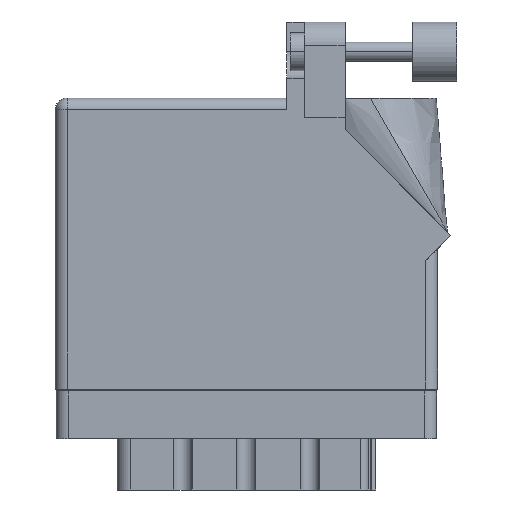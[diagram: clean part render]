
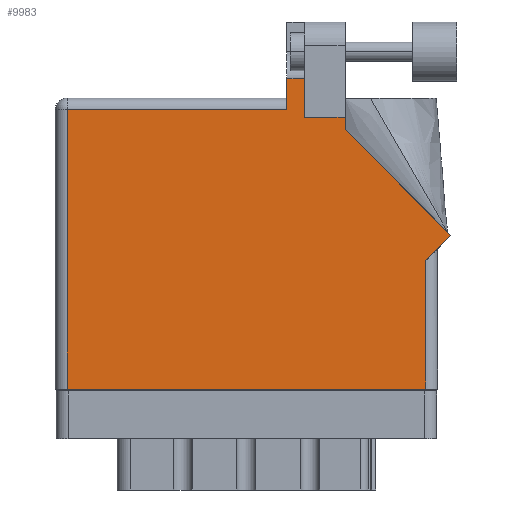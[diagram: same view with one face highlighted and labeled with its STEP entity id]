
A CAD part, front view. The second image highlights one B-rep face of the part: STEP entity #9983.
In plain terms, the highlighted face is planar.
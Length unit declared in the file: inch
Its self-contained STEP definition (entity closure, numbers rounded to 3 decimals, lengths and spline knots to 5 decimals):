
#155 = LINE ( 'NONE', #9917, #4669 ) ;
#1623 = EDGE_CURVE ( 'NONE', #24124, #27353, #11907, .T. ) ;
#1739 = DIRECTION ( 'NONE',  ( -1., 0., 0. ) ) ;
#1949 = CARTESIAN_POINT ( 'NONE',  ( 1.948, 0.675, 0. ) ) ;
#1974 = LINE ( 'NONE', #24542, #31840 ) ;
#2134 = PLANE ( 'NONE',  #11080 ) ;
#3184 = EDGE_CURVE ( 'NONE', #17469, #32814, #34057, .T. ) ;
#3371 = ORIENTED_EDGE ( 'NONE', *, *, #4933, .T. ) ;
#3583 = VECTOR ( 'NONE', #19565, 39.37008 ) ;
#3802 = VERTEX_POINT ( 'NONE', #10859 ) ;
#3973 = DIRECTION ( 'NONE',  ( 0.707, 0.707, 0. ) ) ;
#4469 = VERTEX_POINT ( 'NONE', #26020 ) ;
#4598 = VERTEX_POINT ( 'NONE', #9753 ) ;
#4600 = ORIENTED_EDGE ( 'NONE', *, *, #5607, .T. ) ;
#4647 = FACE_OUTER_BOUND ( 'NONE', #32032, .T. ) ;
#4669 = VECTOR ( 'NONE', #15663, 39.37008 ) ;
#4933 = EDGE_CURVE ( 'NONE', #27353, #31644, #31674, .T. ) ;
#5364 = EDGE_CURVE ( 'NONE', #24194, #23527, #28900, .T. ) ;
#5607 = EDGE_CURVE ( 'NONE', #31644, #24194, #9808, .T. ) ;
#5779 = VECTOR ( 'NONE', #32070, 39.37008 ) ;
#6539 = EDGE_CURVE ( 'NONE', #4469, #24124, #32995, .T. ) ;
#7675 = CARTESIAN_POINT ( 'NONE',  ( 1.948, 0., 0. ) ) ;
#7833 = CARTESIAN_POINT ( 'NONE',  ( 1.524, 1.36442, 0. ) ) ;
#8249 = DIRECTION ( 'NONE',  ( -1., 0., 0. ) ) ;
#8918 = CARTESIAN_POINT ( 'NONE',  ( 2.08071, 0.80771, 0. ) ) ;
#9753 = CARTESIAN_POINT ( 'NONE',  ( 1.311, 1.43, 0. ) ) ;
#9808 = LINE ( 'NONE', #35729, #22561 ) ;
#9860 = ORIENTED_EDGE ( 'NONE', *, *, #5364, .T. ) ;
#9882 = CARTESIAN_POINT ( 'NONE',  ( 1.217, 1.468, 0. ) ) ;
#9917 = CARTESIAN_POINT ( 'NONE',  ( 1.311, 1.43, 0. ) ) ;
#9983 = ADVANCED_FACE ( 'NONE', ( #4647 ), #2134, .F. ) ;
#10069 = EDGE_CURVE ( 'NONE', #3802, #17469, #23673, .T. ) ;
#10307 = CARTESIAN_POINT ( 'NONE',  ( 1.524, 1.36442, 0. ) ) ;
#10434 = DIRECTION ( 'NONE',  ( -1., 0., 0. ) ) ;
#10859 = CARTESIAN_POINT ( 'NONE',  ( 1.311, 1.6315, 0. ) ) ;
#10913 = CARTESIAN_POINT ( 'NONE',  ( 1.948, 0.737, 0. ) ) ;
#11080 = AXIS2_PLACEMENT_3D ( 'NONE', #22373, #34245, #8249 ) ;
#11907 = LINE ( 'NONE', #16875, #28661 ) ;
#12183 = VERTEX_POINT ( 'NONE', #17474 ) ;
#13902 = ORIENTED_EDGE ( 'NONE', *, *, #29931, .T. ) ;
#14815 = ORIENTED_EDGE ( 'NONE', *, *, #30037, .T. ) ;
#15663 = DIRECTION ( 'NONE',  ( 0., 1., 0. ) ) ;
#15686 = CARTESIAN_POINT ( 'NONE',  ( 1.217, 1.53, 0. ) ) ;
#15942 = DIRECTION ( 'NONE',  ( 0., -1., 0. ) ) ;
#16422 = VECTOR ( 'NONE', #15942, 39.37008 ) ;
#16875 = CARTESIAN_POINT ( 'NONE',  ( 0., 0., 0. ) ) ;
#17087 = ORIENTED_EDGE ( 'NONE', *, *, #3184, .T. ) ;
#17469 = VERTEX_POINT ( 'NONE', #37457 ) ;
#17474 = CARTESIAN_POINT ( 'NONE',  ( 1.524, 1.43, 0. ) ) ;
#17751 = VECTOR ( 'NONE', #19656, 39.37008 ) ;
#18363 = LINE ( 'NONE', #33481, #27883 ) ;
#19565 = DIRECTION ( 'NONE',  ( 0., 1., 0. ) ) ;
#19656 = DIRECTION ( 'NONE',  ( 0., 1., 0. ) ) ;
#20331 = VECTOR ( 'NONE', #21116, 39.37008 ) ;
#21116 = DIRECTION ( 'NONE',  ( 0., -1., 0. ) ) ;
#22373 = CARTESIAN_POINT ( 'NONE',  ( 0., 1.53, 0. ) ) ;
#22561 = VECTOR ( 'NONE', #3973, 39.37008 ) ;
#22917 = ORIENTED_EDGE ( 'NONE', *, *, #6539, .T. ) ;
#23527 = VERTEX_POINT ( 'NONE', #10307 ) ;
#23673 = LINE ( 'NONE', #37170, #28205 ) ;
#24124 = VERTEX_POINT ( 'NONE', #33203 ) ;
#24157 = CARTESIAN_POINT ( 'NONE',  ( 0.062, 0., 0. ) ) ;
#24194 = VERTEX_POINT ( 'NONE', #24501 ) ;
#24501 = CARTESIAN_POINT ( 'NONE',  ( 2.08071, 0.80771, 0. ) ) ;
#24542 = CARTESIAN_POINT ( 'NONE',  ( 0., 1.468, 0. ) ) ;
#26020 = CARTESIAN_POINT ( 'NONE',  ( 0.062, 1.468, 0. ) ) ;
#26356 = LINE ( 'NONE', #7833, #17751 ) ;
#27353 = VERTEX_POINT ( 'NONE', #7675 ) ;
#27883 = VECTOR ( 'NONE', #1739, 39.37008 ) ;
#28205 = VECTOR ( 'NONE', #33891, 39.37008 ) ;
#28391 = DIRECTION ( 'NONE',  ( 1., 0., 0. ) ) ;
#28661 = VECTOR ( 'NONE', #28391, 39.37008 ) ;
#28841 = EDGE_CURVE ( 'NONE', #12183, #4598, #18363, .T. ) ;
#28900 = LINE ( 'NONE', #8918, #5779 ) ;
#29931 = EDGE_CURVE ( 'NONE', #4598, #3802, #155, .T. ) ;
#30037 = EDGE_CURVE ( 'NONE', #32814, #4469, #1974, .T. ) ;
#30752 = EDGE_CURVE ( 'NONE', #23527, #12183, #26356, .T. ) ;
#31644 = VERTEX_POINT ( 'NONE', #1949 ) ;
#31674 = LINE ( 'NONE', #10913, #3583 ) ;
#31840 = VECTOR ( 'NONE', #10434, 39.37008 ) ;
#32032 = EDGE_LOOP ( 'NONE', ( #13902, #35831, #17087, #14815, #22917, #33429, #3371, #4600, #9860, #35209, #32572 ) ) ;
#32070 = DIRECTION ( 'NONE',  ( -0.707, 0.707, 0. ) ) ;
#32572 = ORIENTED_EDGE ( 'NONE', *, *, #28841, .T. ) ;
#32814 = VERTEX_POINT ( 'NONE', #9882 ) ;
#32995 = LINE ( 'NONE', #24157, #20331 ) ;
#33203 = CARTESIAN_POINT ( 'NONE',  ( 0.062, 0., 0. ) ) ;
#33429 = ORIENTED_EDGE ( 'NONE', *, *, #1623, .T. ) ;
#33481 = CARTESIAN_POINT ( 'NONE',  ( 1.524, 1.43, 0. ) ) ;
#33891 = DIRECTION ( 'NONE',  ( -1., 0., 0. ) ) ;
#34057 = LINE ( 'NONE', #15686, #16422 ) ;
#34245 = DIRECTION ( 'NONE',  ( 0., 0., -1. ) ) ;
#35209 = ORIENTED_EDGE ( 'NONE', *, *, #30752, .T. ) ;
#35729 = CARTESIAN_POINT ( 'NONE',  ( 2.01, 0.737, 0. ) ) ;
#35831 = ORIENTED_EDGE ( 'NONE', *, *, #10069, .T. ) ;
#37170 = CARTESIAN_POINT ( 'NONE',  ( 1.64177, 1.6315, 0. ) ) ;
#37457 = CARTESIAN_POINT ( 'NONE',  ( 1.217, 1.6315, 0. ) ) ;
